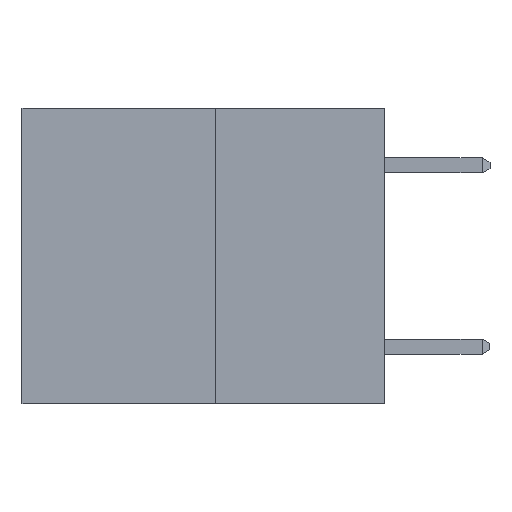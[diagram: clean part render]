
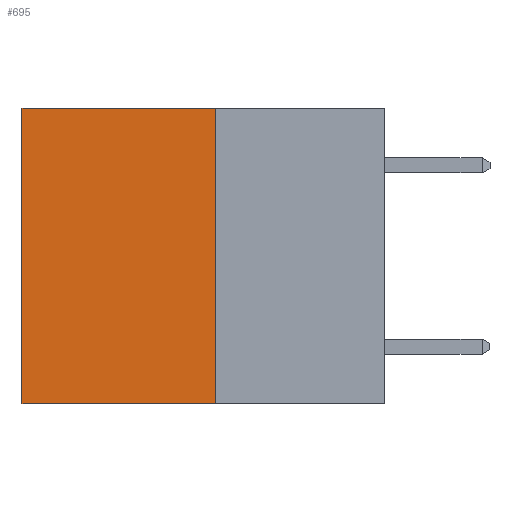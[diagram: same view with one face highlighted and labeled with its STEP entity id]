
A CAD part, left-side view. The second image highlights one B-rep face of the part: STEP entity #695.
In plain terms, the highlighted planar face has unit normal (-1, 0, 0).
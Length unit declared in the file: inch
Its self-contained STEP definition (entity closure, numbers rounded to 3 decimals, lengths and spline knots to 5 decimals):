
#429 = LINE ( 'NONE', #4766, #2700 ) ;
#695 = ADVANCED_FACE ( 'NONE', ( #14638 ), #16487, .F. ) ;
#1293 = ORIENTED_EDGE ( 'NONE', *, *, #4872, .F. ) ;
#1946 = DIRECTION ( 'NONE',  ( 0., 0., -1. ) ) ;
#2700 = VECTOR ( 'NONE', #1946, 39.37008 ) ;
#3017 = CARTESIAN_POINT ( 'NONE',  ( 0.3165, 0.28, 0. ) ) ;
#4295 = VECTOR ( 'NONE', #4435, 39.37008 ) ;
#4435 = DIRECTION ( 'NONE',  ( 0., 1., 0. ) ) ;
#4766 = CARTESIAN_POINT ( 'NONE',  ( 0.3165, 0.28, -0.49 ) ) ;
#4872 = EDGE_CURVE ( 'NONE', #12276, #13348, #429, .T. ) ;
#5142 = LINE ( 'NONE', #17175, #13328 ) ;
#5231 = EDGE_CURVE ( 'NONE', #12276, #8024, #15219, .T. ) ;
#5623 = VERTEX_POINT ( 'NONE', #10537 ) ;
#6162 = CARTESIAN_POINT ( 'NONE',  ( 0.3165, 0.28, -0.49 ) ) ;
#6424 = EDGE_LOOP ( 'NONE', ( #12864, #14264, #1293, #11966 ) ) ;
#6546 = CARTESIAN_POINT ( 'NONE',  ( 0.3165, 0.28, 0. ) ) ;
#6706 = CARTESIAN_POINT ( 'NONE',  ( 0.3165, 0.6, -0.49 ) ) ;
#7760 = DIRECTION ( 'NONE',  ( 0., 0., -1. ) ) ;
#7979 = LINE ( 'NONE', #6706, #8436 ) ;
#8024 = VERTEX_POINT ( 'NONE', #10689 ) ;
#8436 = VECTOR ( 'NONE', #18294, 39.37008 ) ;
#9748 = AXIS2_PLACEMENT_3D ( 'NONE', #6162, #12016, #7760 ) ;
#10537 = CARTESIAN_POINT ( 'NONE',  ( 0.3165, 0.6, -0.49 ) ) ;
#10689 = CARTESIAN_POINT ( 'NONE',  ( 0.3165, 0.6, 0. ) ) ;
#11966 = ORIENTED_EDGE ( 'NONE', *, *, #5231, .T. ) ;
#12016 = DIRECTION ( 'NONE',  ( 1., 0., 0. ) ) ;
#12276 = VERTEX_POINT ( 'NONE', #6546 ) ;
#12864 = ORIENTED_EDGE ( 'NONE', *, *, #17361, .T. ) ;
#13244 = EDGE_CURVE ( 'NONE', #13348, #5623, #5142, .T. ) ;
#13328 = VECTOR ( 'NONE', #15511, 39.37008 ) ;
#13348 = VERTEX_POINT ( 'NONE', #14019 ) ;
#14019 = CARTESIAN_POINT ( 'NONE',  ( 0.3165, 0.28, -0.49 ) ) ;
#14264 = ORIENTED_EDGE ( 'NONE', *, *, #13244, .F. ) ;
#14638 = FACE_OUTER_BOUND ( 'NONE', #6424, .T. ) ;
#15219 = LINE ( 'NONE', #3017, #4295 ) ;
#15511 = DIRECTION ( 'NONE',  ( 0., 1., 0. ) ) ;
#16487 = PLANE ( 'NONE',  #9748 ) ;
#17175 = CARTESIAN_POINT ( 'NONE',  ( 0.3165, 0.28, -0.49 ) ) ;
#17361 = EDGE_CURVE ( 'NONE', #8024, #5623, #7979, .T. ) ;
#18294 = DIRECTION ( 'NONE',  ( 0., 0., -1. ) ) ;
